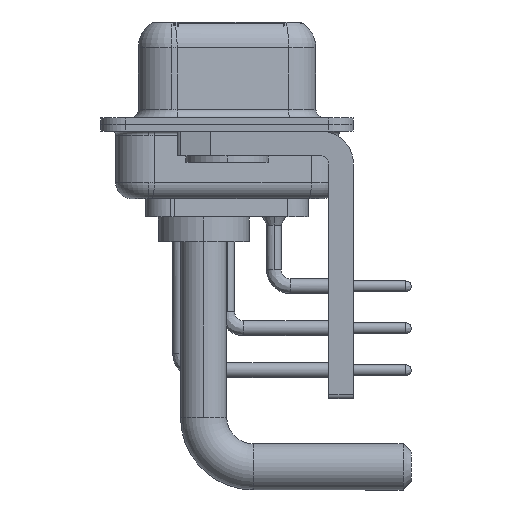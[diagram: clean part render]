
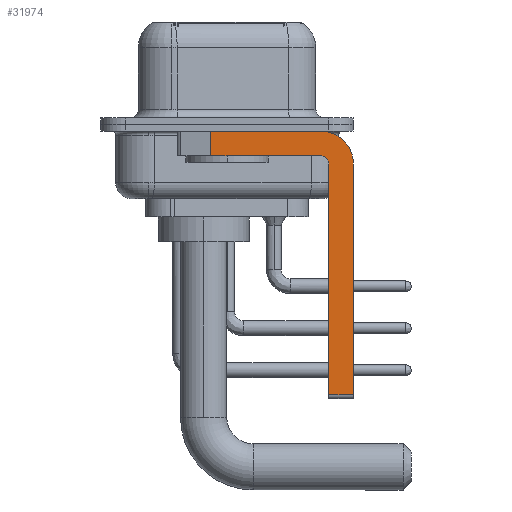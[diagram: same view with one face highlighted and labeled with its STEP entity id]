
A CAD part, left-side view. The second image highlights one B-rep face of the part: STEP entity #31974.
In plain terms, the highlighted planar face has unit normal (-1, 0, 0).
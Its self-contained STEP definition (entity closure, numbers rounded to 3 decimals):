
#165 = VERTEX_POINT ( 'NONE', #25014 ) ;
#208 = VERTEX_POINT ( 'NONE', #32131 ) ;
#426 = VECTOR ( 'NONE', #13563, 1000. ) ;
#737 = EDGE_LOOP ( 'NONE', ( #30748, #5742, #30842, #9404, #26359, #17510, #15285, #19015 ) ) ;
#806 = VERTEX_POINT ( 'NONE', #13142 ) ;
#1612 = AXIS2_PLACEMENT_3D ( 'NONE', #8358, #28899, #16435 ) ;
#2143 = LINE ( 'NONE', #30576, #10308 ) ;
#3341 = CARTESIAN_POINT ( 'NONE',  ( -2.9, 0.978, -1.9 ) ) ;
#3754 = LINE ( 'NONE', #11965, #5759 ) ;
#3757 = CARTESIAN_POINT ( 'NONE',  ( -2.9, 0.978, -1.9 ) ) ;
#3975 = EDGE_CURVE ( 'NONE', #13016, #165, #3754, .T. ) ;
#4596 = DIRECTION ( 'NONE',  ( 0., 0., -1. ) ) ;
#5742 = ORIENTED_EDGE ( 'NONE', *, *, #19623, .T. ) ;
#5759 = VECTOR ( 'NONE', #6423, 1000. ) ;
#6092 = VERTEX_POINT ( 'NONE', #3757 ) ;
#6423 = DIRECTION ( 'NONE',  ( 0., 0., -1. ) ) ;
#7097 = CARTESIAN_POINT ( 'NONE',  ( -2.9, -5.65, -2.4 ) ) ;
#7233 = CARTESIAN_POINT ( 'NONE',  ( -2.9, -7.65, -2.4 ) ) ;
#7482 = EDGE_CURVE ( 'NONE', #11154, #208, #31365, .T. ) ;
#8282 = CARTESIAN_POINT ( 'NONE',  ( -2.9, 3., -0.4 ) ) ;
#8358 = CARTESIAN_POINT ( 'NONE',  ( -2.9, -5.65, -2.4 ) ) ;
#8901 = EDGE_CURVE ( 'NONE', #806, #165, #2143, .T. ) ;
#8955 = CARTESIAN_POINT ( 'NONE',  ( -2.9, 0.978, -0.4 ) ) ;
#9044 = DIRECTION ( 'NONE',  ( -1., 0., 0. ) ) ;
#9344 = CARTESIAN_POINT ( 'NONE',  ( -2.9, -6.15, -2.4 ) ) ;
#9404 = ORIENTED_EDGE ( 'NONE', *, *, #13255, .F. ) ;
#9571 = EDGE_CURVE ( 'NONE', #23646, #6092, #28492, .T. ) ;
#9958 = EDGE_CURVE ( 'NONE', #806, #18245, #15847, .T. ) ;
#10283 = DIRECTION ( 'NONE',  ( 0., 0., 1. ) ) ;
#10308 = VECTOR ( 'NONE', #28197, 1000. ) ;
#11154 = VERTEX_POINT ( 'NONE', #8955 ) ;
#11965 = CARTESIAN_POINT ( 'NONE',  ( -2.9, -7.65, -2.4 ) ) ;
#13016 = VERTEX_POINT ( 'NONE', #7233 ) ;
#13142 = CARTESIAN_POINT ( 'NONE',  ( -2.9, -6.15, -16.35 ) ) ;
#13255 = EDGE_CURVE ( 'NONE', #18245, #23646, #13599, .T. ) ;
#13563 = DIRECTION ( 'NONE',  ( 0., 0., -1. ) ) ;
#13599 = CIRCLE ( 'NONE', #25408, 0.5 ) ;
#13701 = CIRCLE ( 'NONE', #25508, 2. ) ;
#14987 = DIRECTION ( 'NONE',  ( 1., 0., 0. ) ) ;
#15285 = ORIENTED_EDGE ( 'NONE', *, *, #3975, .F. ) ;
#15847 = LINE ( 'NONE', #25915, #25824 ) ;
#15880 = DIRECTION ( 'NONE',  ( 0., 1., 0. ) ) ;
#16435 = DIRECTION ( 'NONE',  ( 0., 0., -1. ) ) ;
#17510 = ORIENTED_EDGE ( 'NONE', *, *, #8901, .T. ) ;
#17870 = CARTESIAN_POINT ( 'NONE',  ( -2.9, -5.65, -1.9 ) ) ;
#18245 = VERTEX_POINT ( 'NONE', #9344 ) ;
#18393 = CARTESIAN_POINT ( 'NONE',  ( -2.9, -5.65, -1.9 ) ) ;
#19015 = ORIENTED_EDGE ( 'NONE', *, *, #28572, .F. ) ;
#19623 = EDGE_CURVE ( 'NONE', #11154, #6092, #26343, .T. ) ;
#21300 = FACE_OUTER_BOUND ( 'NONE', #737, .T. ) ;
#23646 = VERTEX_POINT ( 'NONE', #17870 ) ;
#24978 = DIRECTION ( 'NONE',  ( 0., 0., 1. ) ) ;
#25014 = CARTESIAN_POINT ( 'NONE',  ( -2.9, -7.65, -16.35 ) ) ;
#25265 = VECTOR ( 'NONE', #15880, 1000. ) ;
#25408 = AXIS2_PLACEMENT_3D ( 'NONE', #32141, #9044, #24978 ) ;
#25508 = AXIS2_PLACEMENT_3D ( 'NONE', #7097, #14987, #4596 ) ;
#25824 = VECTOR ( 'NONE', #10283, 1000. ) ;
#25915 = CARTESIAN_POINT ( 'NONE',  ( -2.9, -6.15, -16.6 ) ) ;
#26175 = PLANE ( 'NONE',  #1612 ) ;
#26343 = LINE ( 'NONE', #3341, #426 ) ;
#26359 = ORIENTED_EDGE ( 'NONE', *, *, #9958, .F. ) ;
#28197 = DIRECTION ( 'NONE',  ( 0., -1., 0. ) ) ;
#28492 = LINE ( 'NONE', #18393, #25265 ) ;
#28572 = EDGE_CURVE ( 'NONE', #208, #13016, #13701, .T. ) ;
#28821 = DIRECTION ( 'NONE',  ( 0., -1., 0. ) ) ;
#28842 = VECTOR ( 'NONE', #28821, 1000. ) ;
#28899 = DIRECTION ( 'NONE',  ( 1., 0., 0. ) ) ;
#30576 = CARTESIAN_POINT ( 'NONE',  ( -2.9, -5.65, -16.35 ) ) ;
#30748 = ORIENTED_EDGE ( 'NONE', *, *, #7482, .F. ) ;
#30842 = ORIENTED_EDGE ( 'NONE', *, *, #9571, .F. ) ;
#31365 = LINE ( 'NONE', #8282, #28842 ) ;
#31974 = ADVANCED_FACE ( 'NONE', ( #21300 ), #26175, .F. ) ;
#32131 = CARTESIAN_POINT ( 'NONE',  ( -2.9, -5.65, -0.4 ) ) ;
#32141 = CARTESIAN_POINT ( 'NONE',  ( -2.9, -5.65, -2.4 ) ) ;
